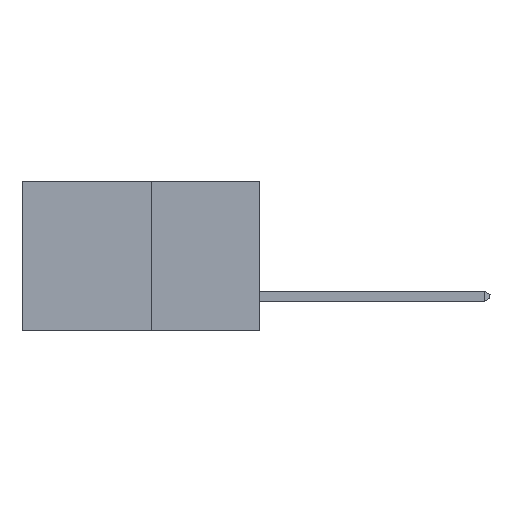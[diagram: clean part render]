
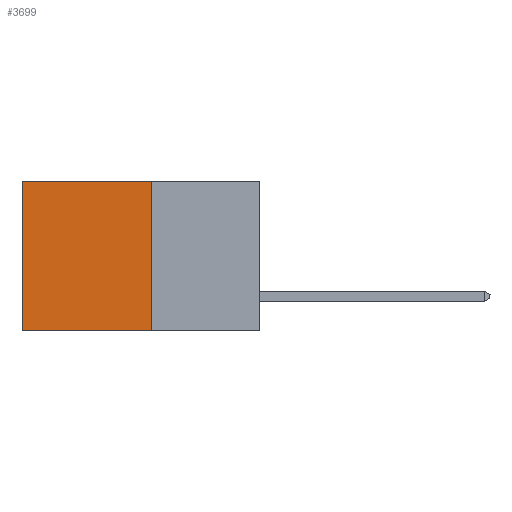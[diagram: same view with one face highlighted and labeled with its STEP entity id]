
A CAD part, left-side view. The second image highlights one B-rep face of the part: STEP entity #3699.
In plain terms, the highlighted planar face has unit normal (-1, 0, 0).
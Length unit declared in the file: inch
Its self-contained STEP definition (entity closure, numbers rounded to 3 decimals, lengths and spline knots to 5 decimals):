
#84 = VERTEX_POINT ( 'NONE', #8099 ) ;
#418 = CARTESIAN_POINT ( 'NONE',  ( 0.277, 0.27, 0. ) ) ;
#706 = EDGE_LOOP ( 'NONE', ( #2097, #8507, #4572, #10657 ) ) ;
#1237 = EDGE_CURVE ( 'NONE', #1277, #11023, #3492, .T. ) ;
#1277 = VERTEX_POINT ( 'NONE', #418 ) ;
#1949 = DIRECTION ( 'NONE',  ( 0., 1., 0. ) ) ;
#2037 = CARTESIAN_POINT ( 'NONE',  ( 0.277, 0.59, 0. ) ) ;
#2097 = ORIENTED_EDGE ( 'NONE', *, *, #9080, .T. ) ;
#2148 = FACE_OUTER_BOUND ( 'NONE', #706, .T. ) ;
#2592 = CARTESIAN_POINT ( 'NONE',  ( 0.277, 0.27, -0.37 ) ) ;
#3019 = CARTESIAN_POINT ( 'NONE',  ( 0.277, 0.27, -0.37 ) ) ;
#3492 = LINE ( 'NONE', #9228, #5623 ) ;
#3699 = ADVANCED_FACE ( 'NONE', ( #2148 ), #7760, .F. ) ;
#4140 = LINE ( 'NONE', #5684, #10703 ) ;
#4572 = ORIENTED_EDGE ( 'NONE', *, *, #4868, .F. ) ;
#4694 = VECTOR ( 'NONE', #1949, 39.37008 ) ;
#4868 = EDGE_CURVE ( 'NONE', #1277, #9014, #4140, .T. ) ;
#5623 = VECTOR ( 'NONE', #7859, 39.37008 ) ;
#5684 = CARTESIAN_POINT ( 'NONE',  ( 0.277, 0.27, -0.37 ) ) ;
#6206 = EDGE_CURVE ( 'NONE', #9014, #84, #9232, .T. ) ;
#6950 = VECTOR ( 'NONE', #11278, 39.37008 ) ;
#7760 = PLANE ( 'NONE',  #9843 ) ;
#7808 = DIRECTION ( 'NONE',  ( 1., 0., 0. ) ) ;
#7859 = DIRECTION ( 'NONE',  ( 0., 1., 0. ) ) ;
#7899 = CARTESIAN_POINT ( 'NONE',  ( 0.277, 0.59, -0.37 ) ) ;
#8051 = DIRECTION ( 'NONE',  ( 0., 0., -1. ) ) ;
#8099 = CARTESIAN_POINT ( 'NONE',  ( 0.277, 0.59, -0.37 ) ) ;
#8507 = ORIENTED_EDGE ( 'NONE', *, *, #6206, .F. ) ;
#9014 = VERTEX_POINT ( 'NONE', #10329 ) ;
#9080 = EDGE_CURVE ( 'NONE', #11023, #84, #9182, .T. ) ;
#9182 = LINE ( 'NONE', #7899, #6950 ) ;
#9228 = CARTESIAN_POINT ( 'NONE',  ( 0.277, 0.27, 0. ) ) ;
#9232 = LINE ( 'NONE', #2592, #4694 ) ;
#9843 = AXIS2_PLACEMENT_3D ( 'NONE', #3019, #7808, #8051 ) ;
#10329 = CARTESIAN_POINT ( 'NONE',  ( 0.277, 0.27, -0.37 ) ) ;
#10617 = DIRECTION ( 'NONE',  ( 0., 0., -1. ) ) ;
#10657 = ORIENTED_EDGE ( 'NONE', *, *, #1237, .T. ) ;
#10703 = VECTOR ( 'NONE', #10617, 39.37008 ) ;
#11023 = VERTEX_POINT ( 'NONE', #2037 ) ;
#11278 = DIRECTION ( 'NONE',  ( 0., 0., -1. ) ) ;
